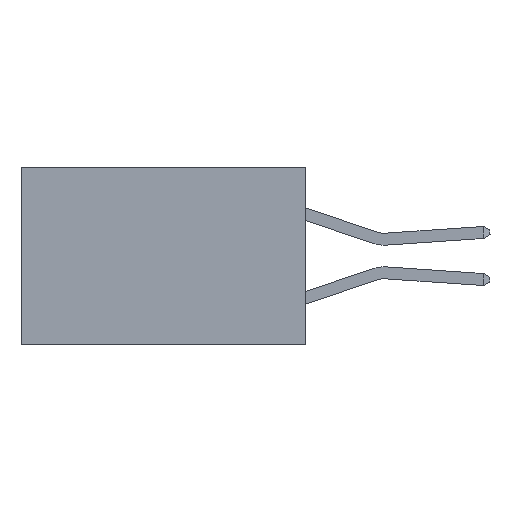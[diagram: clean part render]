
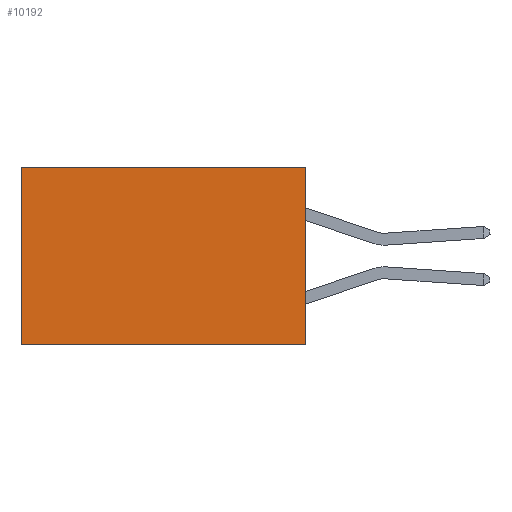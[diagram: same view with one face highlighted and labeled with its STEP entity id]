
A CAD part, left-side view. The second image highlights one B-rep face of the part: STEP entity #10192.
In plain terms, the highlighted planar face has unit normal (-1, 0, 0).
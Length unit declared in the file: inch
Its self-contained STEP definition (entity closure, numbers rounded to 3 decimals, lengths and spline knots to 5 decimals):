
#278 = CARTESIAN_POINT ( 'NONE',  ( 0.277, 0., -0.37 ) ) ;
#552 = VERTEX_POINT ( 'NONE', #4048 ) ;
#1175 = LINE ( 'NONE', #2160, #13274 ) ;
#1327 = CARTESIAN_POINT ( 'NONE',  ( 0.277, 0.59, -0.37 ) ) ;
#1889 = DIRECTION ( 'NONE',  ( 0., 0., -1. ) ) ;
#2160 = CARTESIAN_POINT ( 'NONE',  ( 0.277, 0.59, -0.37 ) ) ;
#2422 = CARTESIAN_POINT ( 'NONE',  ( 0.277, 0., 0. ) ) ;
#2477 = DIRECTION ( 'NONE',  ( 0., 1., 0. ) ) ;
#3403 = VERTEX_POINT ( 'NONE', #13117 ) ;
#3709 = EDGE_LOOP ( 'NONE', ( #12494, #13981, #10865, #6700 ) ) ;
#3898 = EDGE_CURVE ( 'NONE', #9793, #14455, #1175, .T. ) ;
#4048 = CARTESIAN_POINT ( 'NONE',  ( 0.277, 0., -0.37 ) ) ;
#4195 = EDGE_CURVE ( 'NONE', #3403, #9793, #9942, .T. ) ;
#5223 = CARTESIAN_POINT ( 'NONE',  ( 0.277, 0., -0.37 ) ) ;
#5503 = DIRECTION ( 'NONE',  ( 0., 0., -1. ) ) ;
#6110 = VECTOR ( 'NONE', #9217, 39.37008 ) ;
#6687 = CARTESIAN_POINT ( 'NONE',  ( 0.277, 0.59, 0. ) ) ;
#6700 = ORIENTED_EDGE ( 'NONE', *, *, #4195, .T. ) ;
#7798 = DIRECTION ( 'NONE',  ( 0., 1., 0. ) ) ;
#8372 = LINE ( 'NONE', #5223, #14307 ) ;
#9217 = DIRECTION ( 'NONE',  ( 0., 0., -1. ) ) ;
#9793 = VERTEX_POINT ( 'NONE', #6687 ) ;
#9942 = LINE ( 'NONE', #2422, #12686 ) ;
#10192 = ADVANCED_FACE ( 'NONE', ( #13819 ), #10444, .F. ) ;
#10444 = PLANE ( 'NONE',  #14646 ) ;
#10865 = ORIENTED_EDGE ( 'NONE', *, *, #15094, .F. ) ;
#12494 = ORIENTED_EDGE ( 'NONE', *, *, #3898, .T. ) ;
#12650 = EDGE_CURVE ( 'NONE', #552, #14455, #8372, .T. ) ;
#12686 = VECTOR ( 'NONE', #2477, 39.37008 ) ;
#12800 = DIRECTION ( 'NONE',  ( 1., 0., 0. ) ) ;
#13117 = CARTESIAN_POINT ( 'NONE',  ( 0.277, 0., 0. ) ) ;
#13274 = VECTOR ( 'NONE', #1889, 39.37008 ) ;
#13819 = FACE_OUTER_BOUND ( 'NONE', #3709, .T. ) ;
#13939 = CARTESIAN_POINT ( 'NONE',  ( 0.277, 0., -0.37 ) ) ;
#13981 = ORIENTED_EDGE ( 'NONE', *, *, #12650, .F. ) ;
#14307 = VECTOR ( 'NONE', #7798, 39.37008 ) ;
#14455 = VERTEX_POINT ( 'NONE', #1327 ) ;
#14646 = AXIS2_PLACEMENT_3D ( 'NONE', #13939, #12800, #5503 ) ;
#15094 = EDGE_CURVE ( 'NONE', #3403, #552, #15656, .T. ) ;
#15656 = LINE ( 'NONE', #278, #6110 ) ;
